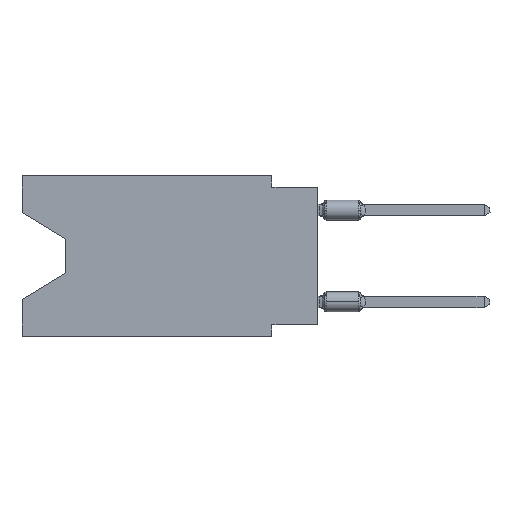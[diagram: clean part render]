
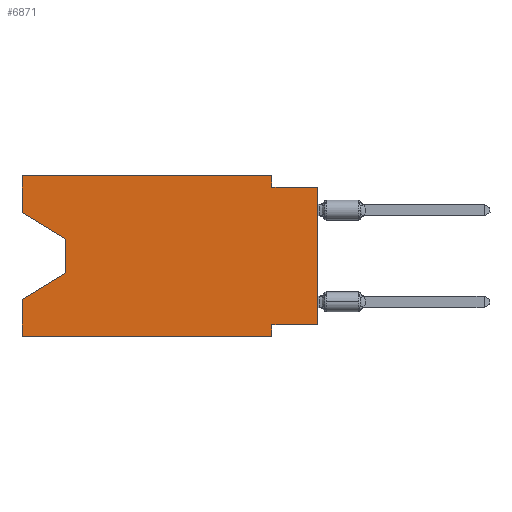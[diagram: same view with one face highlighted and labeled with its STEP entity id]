
A CAD part, left-side view. The second image highlights one B-rep face of the part: STEP entity #6871.
In plain terms, the highlighted planar face has unit normal (-1, 0, 0).
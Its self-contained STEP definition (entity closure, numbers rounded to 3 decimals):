
#260 = VERTEX_POINT ( 'NONE', #13653 ) ;
#265 = DIRECTION ( 'NONE',  ( 0., 0., 1. ) ) ;
#667 = DIRECTION ( 'NONE',  ( 0., 0., -1. ) ) ;
#794 = ORIENTED_EDGE ( 'NONE', *, *, #6616, .T. ) ;
#953 = ORIENTED_EDGE ( 'NONE', *, *, #13910, .T. ) ;
#1235 = ORIENTED_EDGE ( 'NONE', *, *, #1898, .F. ) ;
#1332 = VECTOR ( 'NONE', #8298, 1000. ) ;
#1356 = DIRECTION ( 'NONE',  ( 0., 0.855, -0.519 ) ) ;
#1601 = CARTESIAN_POINT ( 'NONE',  ( 0., 2.54, -8.89 ) ) ;
#1898 = EDGE_CURVE ( 'NONE', #8925, #12886, #10447, .T. ) ;
#1917 = ORIENTED_EDGE ( 'NONE', *, *, #8485, .F. ) ;
#2020 = DIRECTION ( 'NONE',  ( 0., -1., 0. ) ) ;
#2111 = LINE ( 'NONE', #6761, #4562 ) ;
#2386 = EDGE_CURVE ( 'NONE', #9340, #5862, #11856, .T. ) ;
#2559 = CARTESIAN_POINT ( 'NONE',  ( 0., 16.383, 0. ) ) ;
#2925 = ORIENTED_EDGE ( 'NONE', *, *, #14189, .T. ) ;
#3057 = DIRECTION ( 'NONE',  ( 0., 1., 0. ) ) ;
#3236 = CARTESIAN_POINT ( 'NONE',  ( 0., 16.383, 0. ) ) ;
#3279 = CARTESIAN_POINT ( 'NONE',  ( 0., 2.54, -8.255 ) ) ;
#3299 = VECTOR ( 'NONE', #3763, 1000. ) ;
#3365 = EDGE_CURVE ( 'NONE', #7672, #4866, #14436, .T. ) ;
#3416 = CARTESIAN_POINT ( 'NONE',  ( 0., 2.54, 0. ) ) ;
#3427 = CARTESIAN_POINT ( 'NONE',  ( 0., 13.97, -3.505 ) ) ;
#3496 = LINE ( 'NONE', #13991, #5943 ) ;
#3535 = DIRECTION ( 'NONE',  ( 0., 0., 1. ) ) ;
#3591 = VECTOR ( 'NONE', #2020, 1000. ) ;
#3763 = DIRECTION ( 'NONE',  ( 0., -0.855, -0.519 ) ) ;
#3806 = CARTESIAN_POINT ( 'NONE',  ( 0., 16.383, -8.89 ) ) ;
#3815 = VERTEX_POINT ( 'NONE', #10913 ) ;
#4195 = CARTESIAN_POINT ( 'NONE',  ( 0., 0., -0.635 ) ) ;
#4358 = LINE ( 'NONE', #13473, #13441 ) ;
#4360 = VERTEX_POINT ( 'NONE', #3427 ) ;
#4562 = VECTOR ( 'NONE', #11387, 1000. ) ;
#4790 = CARTESIAN_POINT ( 'NONE',  ( 0., 2.54, -8.89 ) ) ;
#4866 = VERTEX_POINT ( 'NONE', #5540 ) ;
#5235 = CARTESIAN_POINT ( 'NONE',  ( 0., 2.54, 0. ) ) ;
#5415 = VERTEX_POINT ( 'NONE', #10676 ) ;
#5511 = ORIENTED_EDGE ( 'NONE', *, *, #10168, .T. ) ;
#5540 = CARTESIAN_POINT ( 'NONE',  ( 0., 2.54, -0.635 ) ) ;
#5862 = VERTEX_POINT ( 'NONE', #1601 ) ;
#5943 = VECTOR ( 'NONE', #6860, 1000. ) ;
#6131 = LINE ( 'NONE', #2559, #8457 ) ;
#6236 = AXIS2_PLACEMENT_3D ( 'NONE', #7950, #9989, #12558 ) ;
#6449 = LINE ( 'NONE', #14811, #13978 ) ;
#6616 = EDGE_CURVE ( 'NONE', #8925, #4360, #6974, .T. ) ;
#6761 = CARTESIAN_POINT ( 'NONE',  ( 0., 0., 0. ) ) ;
#6860 = DIRECTION ( 'NONE',  ( 0., -1., 0. ) ) ;
#6871 = ADVANCED_FACE ( 'NONE', ( #13572 ), #9080, .F. ) ;
#6974 = LINE ( 'NONE', #10519, #3299 ) ;
#7241 = VECTOR ( 'NONE', #667, 1000. ) ;
#7303 = VERTEX_POINT ( 'NONE', #4195 ) ;
#7672 = VERTEX_POINT ( 'NONE', #3416 ) ;
#7950 = CARTESIAN_POINT ( 'NONE',  ( 0., 16.383, 0. ) ) ;
#8287 = ORIENTED_EDGE ( 'NONE', *, *, #3365, .F. ) ;
#8298 = DIRECTION ( 'NONE',  ( 0., -1., 0. ) ) ;
#8299 = DIRECTION ( 'NONE',  ( 0., 0., -1. ) ) ;
#8352 = CARTESIAN_POINT ( 'NONE',  ( 0., 13.97, -5.385 ) ) ;
#8457 = VECTOR ( 'NONE', #265, 1000. ) ;
#8485 = EDGE_CURVE ( 'NONE', #5415, #9340, #4358, .T. ) ;
#8561 = ORIENTED_EDGE ( 'NONE', *, *, #9498, .T. ) ;
#8804 = EDGE_LOOP ( 'NONE', ( #794, #5511, #953, #11280, #8561, #10208, #1917, #2925, #12627, #8287, #9502, #1235 ) ) ;
#8925 = VERTEX_POINT ( 'NONE', #9154 ) ;
#9080 = PLANE ( 'NONE',  #6236 ) ;
#9154 = CARTESIAN_POINT ( 'NONE',  ( 0., 16.383, -2.038 ) ) ;
#9340 = VERTEX_POINT ( 'NONE', #3279 ) ;
#9498 = EDGE_CURVE ( 'NONE', #13480, #5862, #14075, .T. ) ;
#9502 = ORIENTED_EDGE ( 'NONE', *, *, #14383, .F. ) ;
#9575 = EDGE_CURVE ( 'NONE', #4866, #7303, #3496, .T. ) ;
#9643 = LINE ( 'NONE', #8352, #10611 ) ;
#9989 = DIRECTION ( 'NONE',  ( 1., 0., 0. ) ) ;
#9994 = LINE ( 'NONE', #13418, #3591 ) ;
#10149 = VECTOR ( 'NONE', #3535, 1000. ) ;
#10168 = EDGE_CURVE ( 'NONE', #4360, #260, #6449, .T. ) ;
#10208 = ORIENTED_EDGE ( 'NONE', *, *, #2386, .F. ) ;
#10447 = LINE ( 'NONE', #3236, #10149 ) ;
#10519 = CARTESIAN_POINT ( 'NONE',  ( 0., 16.383, -2.038 ) ) ;
#10611 = VECTOR ( 'NONE', #1356, 1000. ) ;
#10676 = CARTESIAN_POINT ( 'NONE',  ( 0., 0., -8.255 ) ) ;
#10913 = CARTESIAN_POINT ( 'NONE',  ( 0., 16.383, -6.852 ) ) ;
#11280 = ORIENTED_EDGE ( 'NONE', *, *, #14245, .F. ) ;
#11298 = DIRECTION ( 'NONE',  ( 0., 0., -1. ) ) ;
#11364 = VECTOR ( 'NONE', #8299, 1000. ) ;
#11387 = DIRECTION ( 'NONE',  ( 0., 0., 1. ) ) ;
#11856 = LINE ( 'NONE', #4790, #11364 ) ;
#12558 = DIRECTION ( 'NONE',  ( 0., 0., -1. ) ) ;
#12614 = CARTESIAN_POINT ( 'NONE',  ( 0., 16.383, -8.89 ) ) ;
#12627 = ORIENTED_EDGE ( 'NONE', *, *, #9575, .F. ) ;
#12886 = VERTEX_POINT ( 'NONE', #12938 ) ;
#12938 = CARTESIAN_POINT ( 'NONE',  ( 0., 16.383, 0. ) ) ;
#13418 = CARTESIAN_POINT ( 'NONE',  ( 0., 16.383, 0. ) ) ;
#13441 = VECTOR ( 'NONE', #3057, 1000. ) ;
#13473 = CARTESIAN_POINT ( 'NONE',  ( 0., 0., -8.255 ) ) ;
#13480 = VERTEX_POINT ( 'NONE', #3806 ) ;
#13572 = FACE_OUTER_BOUND ( 'NONE', #8804, .T. ) ;
#13653 = CARTESIAN_POINT ( 'NONE',  ( 0., 13.97, -5.385 ) ) ;
#13910 = EDGE_CURVE ( 'NONE', #260, #3815, #9643, .T. ) ;
#13978 = VECTOR ( 'NONE', #11298, 1000. ) ;
#13991 = CARTESIAN_POINT ( 'NONE',  ( 0., 0., -0.635 ) ) ;
#14075 = LINE ( 'NONE', #12614, #1332 ) ;
#14189 = EDGE_CURVE ( 'NONE', #5415, #7303, #2111, .T. ) ;
#14245 = EDGE_CURVE ( 'NONE', #13480, #3815, #6131, .T. ) ;
#14383 = EDGE_CURVE ( 'NONE', #12886, #7672, #9994, .T. ) ;
#14436 = LINE ( 'NONE', #5235, #7241 ) ;
#14811 = CARTESIAN_POINT ( 'NONE',  ( 0., 13.97, -3.505 ) ) ;
